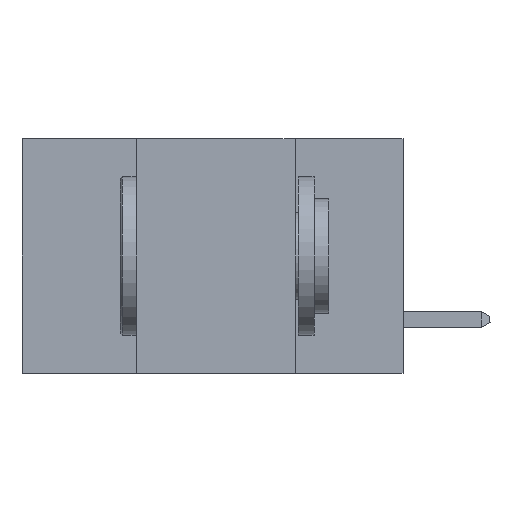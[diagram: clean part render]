
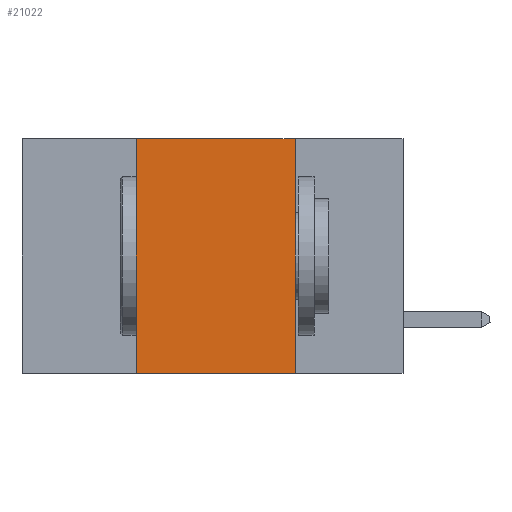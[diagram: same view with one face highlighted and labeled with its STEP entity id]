
A CAD part, left-side view. The second image highlights one B-rep face of the part: STEP entity #21022.
In plain terms, the highlighted planar face has unit normal (-1, 0, 0).
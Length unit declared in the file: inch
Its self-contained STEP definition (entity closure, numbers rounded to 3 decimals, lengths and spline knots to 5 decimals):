
#300 = VERTEX_POINT ( 'NONE', #14510 ) ;
#637 = VECTOR ( 'NONE', #5846, 39.37008 ) ;
#791 = CARTESIAN_POINT ( 'NONE',  ( 0., 0.42, 0. ) ) ;
#840 = CARTESIAN_POINT ( 'NONE',  ( 0., 0.6, -0.37 ) ) ;
#2633 = ORIENTED_EDGE ( 'NONE', *, *, #7163, .F. ) ;
#5066 = EDGE_LOOP ( 'NONE', ( #21277, #13130, #2633, #5400 ) ) ;
#5306 = DIRECTION ( 'NONE',  ( 0., 0., -1. ) ) ;
#5400 = ORIENTED_EDGE ( 'NONE', *, *, #21842, .T. ) ;
#5698 = LINE ( 'NONE', #840, #20361 ) ;
#5846 = DIRECTION ( 'NONE',  ( 0., 0., 1. ) ) ;
#6549 = LINE ( 'NONE', #8569, #21742 ) ;
#7163 = EDGE_CURVE ( 'NONE', #10915, #17056, #22118, .T. ) ;
#7453 = CARTESIAN_POINT ( 'NONE',  ( 0., 0.42, 0. ) ) ;
#8569 = CARTESIAN_POINT ( 'NONE',  ( 0., 0.6, 0. ) ) ;
#9232 = CARTESIAN_POINT ( 'NONE',  ( 0., 0.17, 0. ) ) ;
#9989 = VECTOR ( 'NONE', #17948, 39.37008 ) ;
#10143 = DIRECTION ( 'NONE',  ( 0., -1., 0. ) ) ;
#10410 = DIRECTION ( 'NONE',  ( 1., 0., 0. ) ) ;
#10915 = VERTEX_POINT ( 'NONE', #15611 ) ;
#11047 = CARTESIAN_POINT ( 'NONE',  ( 0., 0.17, -0.37 ) ) ;
#11222 = DIRECTION ( 'NONE',  ( 0., -1., 0. ) ) ;
#12155 = CARTESIAN_POINT ( 'NONE',  ( 0., 0.6, 0. ) ) ;
#12686 = AXIS2_PLACEMENT_3D ( 'NONE', #12155, #10410, #5306 ) ;
#13130 = ORIENTED_EDGE ( 'NONE', *, *, #17465, .F. ) ;
#14510 = CARTESIAN_POINT ( 'NONE',  ( 0., 0.17, 0. ) ) ;
#15611 = CARTESIAN_POINT ( 'NONE',  ( 0., 0.42, -0.37 ) ) ;
#17056 = VERTEX_POINT ( 'NONE', #7453 ) ;
#17312 = PLANE ( 'NONE',  #12686 ) ;
#17465 = EDGE_CURVE ( 'NONE', #17056, #300, #6549, .T. ) ;
#17651 = EDGE_CURVE ( 'NONE', #300, #20666, #20035, .T. ) ;
#17948 = DIRECTION ( 'NONE',  ( 0., 0., -1. ) ) ;
#20035 = LINE ( 'NONE', #9232, #9989 ) ;
#20361 = VECTOR ( 'NONE', #11222, 39.37008 ) ;
#20408 = FACE_OUTER_BOUND ( 'NONE', #5066, .T. ) ;
#20666 = VERTEX_POINT ( 'NONE', #11047 ) ;
#21022 = ADVANCED_FACE ( 'NONE', ( #20408 ), #17312, .F. ) ;
#21277 = ORIENTED_EDGE ( 'NONE', *, *, #17651, .F. ) ;
#21742 = VECTOR ( 'NONE', #10143, 39.37008 ) ;
#21842 = EDGE_CURVE ( 'NONE', #10915, #20666, #5698, .T. ) ;
#22118 = LINE ( 'NONE', #791, #637 ) ;
